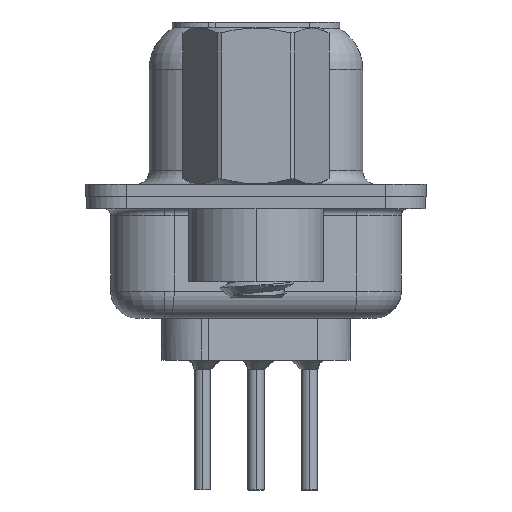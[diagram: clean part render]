
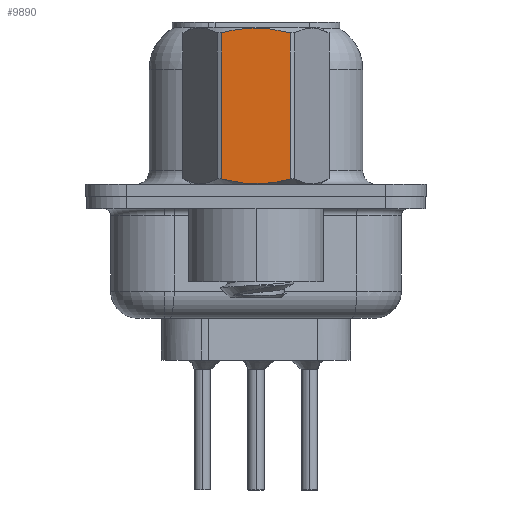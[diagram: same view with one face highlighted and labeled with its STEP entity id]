
A CAD part, left-side view. The second image highlights one B-rep face of the part: STEP entity #9890.
In plain terms, the highlighted planar face has unit normal (-1, 0, 0).
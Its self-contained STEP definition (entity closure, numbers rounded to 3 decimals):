
#626 = CARTESIAN_POINT ( 'NONE',  ( -2.381, -0.432, 0.485 ) ) ;
#802 = CARTESIAN_POINT ( 'NONE',  ( -2.381, -1.273, 3.792 ) ) ;
#2176 = CARTESIAN_POINT ( 'NONE',  ( -2.381, 1.065, 6.104 ) ) ;
#3191 = CARTESIAN_POINT ( 'NONE',  ( -2.381, -1.066, 0.596 ) ) ;
#3385 = ORIENTED_EDGE ( 'NONE', *, *, #22619, .T. ) ;
#4197 = CARTESIAN_POINT ( 'NONE',  ( -2.381, -1.273, 0.652 ) ) ;
#6461 = CARTESIAN_POINT ( 'NONE',  ( -2.381, 1.273, 6.048 ) ) ;
#8077 = CARTESIAN_POINT ( 'NONE',  ( -2.381, 1.273, 0.652 ) ) ;
#8194 = CARTESIAN_POINT ( 'NONE',  ( -2.381, 1.065, 0.596 ) ) ;
#9574 = VERTEX_POINT ( 'NONE', #4197 ) ;
#9890 = ADVANCED_FACE ( 'NONE', ( #20248 ), #20991, .T. ) ;
#10010 = CARTESIAN_POINT ( 'NONE',  ( -2.381, 1.273, 3.792 ) ) ;
#10675 = B_SPLINE_CURVE_WITH_KNOTS ( 'NONE', 3,
 ( #14773, #25168, #27799, #12275, #30355, #14888, #32975, #17489, #2176, #20100 ),
 .UNSPECIFIED., .F., .F.,
 ( 4, 2, 2, 2, 4 ),
 ( 0.001, 0.002, 0.002, 0.003, 0.004 ),
 .UNSPECIFIED. ) ;
#10733 = VERTEX_POINT ( 'NONE', #29979 ) ;
#10840 = DIRECTION ( 'NONE',  ( -1., 0., 0. ) ) ;
#11037 = DIRECTION ( 'NONE',  ( 0., 0., 1. ) ) ;
#12275 = CARTESIAN_POINT ( 'NONE',  ( -2.381, -0.432, 6.215 ) ) ;
#12554 = DIRECTION ( 'NONE',  ( 0., 0., -1. ) ) ;
#13275 = EDGE_CURVE ( 'NONE', #15662, #9574, #23694, .T. ) ;
#13307 = CARTESIAN_POINT ( 'NONE',  ( -2.381, 0.428, 0.485 ) ) ;
#14569 = EDGE_CURVE ( 'NONE', #10733, #22420, #10675, .T. ) ;
#14773 = CARTESIAN_POINT ( 'NONE',  ( -2.381, -1.273, 6.048 ) ) ;
#14888 = CARTESIAN_POINT ( 'NONE',  ( -2.381, 0.215, 6.232 ) ) ;
#15662 = VERTEX_POINT ( 'NONE', #27484 ) ;
#15753 = LINE ( 'NONE', #10010, #27903 ) ;
#15932 = CARTESIAN_POINT ( 'NONE',  ( -2.381, -0.215, 0.468 ) ) ;
#17489 = CARTESIAN_POINT ( 'NONE',  ( -2.381, 0.853, 6.151 ) ) ;
#17586 = LINE ( 'NONE', #802, #22007 ) ;
#18490 = CARTESIAN_POINT ( 'NONE',  ( -2.381, -0.858, 0.55 ) ) ;
#20100 = CARTESIAN_POINT ( 'NONE',  ( -2.381, 1.273, 6.048 ) ) ;
#20248 = FACE_OUTER_BOUND ( 'NONE', #29558, .T. ) ;
#20991 = PLANE ( 'NONE',  #30068 ) ;
#21113 = CARTESIAN_POINT ( 'NONE',  ( -2.381, -1.273, 0.652 ) ) ;
#22007 = VECTOR ( 'NONE', #11037, 1000. ) ;
#22420 = VERTEX_POINT ( 'NONE', #6461 ) ;
#22619 = EDGE_CURVE ( 'NONE', #22420, #15662, #15753, .T. ) ;
#23694 = B_SPLINE_CURVE_WITH_KNOTS ( 'NONE', 3,
 ( #8077, #8194, #28786, #13307, #31395, #15932, #626, #18490, #3191, #21113 ),
 .UNSPECIFIED., .F., .F.,
 ( 4, 2, 2, 2, 4 ),
 ( 0.003, 0.003, 0.004, 0.004, 0.005 ),
 .UNSPECIFIED. ) ;
#24496 = ORIENTED_EDGE ( 'NONE', *, *, #13275, .T. ) ;
#25168 = CARTESIAN_POINT ( 'NONE',  ( -2.381, -1.066, 6.104 ) ) ;
#26322 = CARTESIAN_POINT ( 'NONE',  ( -2.381, 1.375, -3.75 ) ) ;
#27484 = CARTESIAN_POINT ( 'NONE',  ( -2.381, 1.273, 0.652 ) ) ;
#27799 = CARTESIAN_POINT ( 'NONE',  ( -2.381, -0.858, 6.15 ) ) ;
#27903 = VECTOR ( 'NONE', #12554, 1000. ) ;
#28234 = EDGE_CURVE ( 'NONE', #9574, #10733, #17586, .T. ) ;
#28786 = CARTESIAN_POINT ( 'NONE',  ( -2.381, 0.853, 0.549 ) ) ;
#28889 = DIRECTION ( 'NONE',  ( 0., -1., 0. ) ) ;
#29558 = EDGE_LOOP ( 'NONE', ( #24496, #31340, #30922, #3385 ) ) ;
#29979 = CARTESIAN_POINT ( 'NONE',  ( -2.381, -1.273, 6.048 ) ) ;
#30068 = AXIS2_PLACEMENT_3D ( 'NONE', #26322, #10840, #28889 ) ;
#30355 = CARTESIAN_POINT ( 'NONE',  ( -2.381, -0.215, 6.232 ) ) ;
#30922 = ORIENTED_EDGE ( 'NONE', *, *, #14569, .T. ) ;
#31340 = ORIENTED_EDGE ( 'NONE', *, *, #28234, .T. ) ;
#31395 = CARTESIAN_POINT ( 'NONE',  ( -2.381, 0.215, 0.468 ) ) ;
#32975 = CARTESIAN_POINT ( 'NONE',  ( -2.381, 0.428, 6.215 ) ) ;
